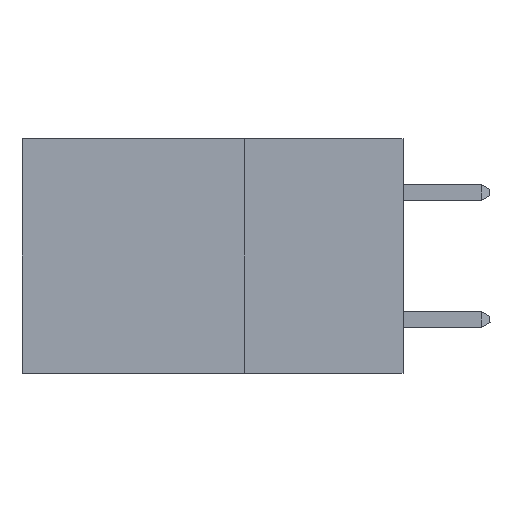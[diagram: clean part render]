
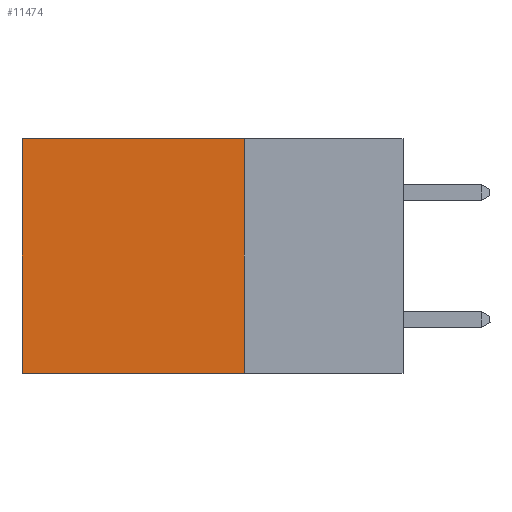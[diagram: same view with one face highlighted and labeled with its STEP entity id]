
A CAD part, left-side view. The second image highlights one B-rep face of the part: STEP entity #11474.
In plain terms, the highlighted planar face has unit normal (-1, 0, 0).
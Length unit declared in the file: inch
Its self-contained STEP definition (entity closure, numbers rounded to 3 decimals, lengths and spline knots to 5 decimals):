
#1245 = LINE ( 'NONE', #22937, #1663 ) ;
#1663 = VECTOR ( 'NONE', #23508, 39.37008 ) ;
#2475 = DIRECTION ( 'NONE',  ( 1., 0., 0. ) ) ;
#2815 = ORIENTED_EDGE ( 'NONE', *, *, #31033, .F. ) ;
#3150 = VECTOR ( 'NONE', #25215, 39.37008 ) ;
#3590 = VERTEX_POINT ( 'NONE', #11174 ) ;
#4204 = FACE_OUTER_BOUND ( 'NONE', #9429, .T. ) ;
#6728 = CARTESIAN_POINT ( 'NONE',  ( 0.2875, 0.25, -0.37 ) ) ;
#9253 = LINE ( 'NONE', #25268, #23292 ) ;
#9429 = EDGE_LOOP ( 'NONE', ( #11271, #14414, #2815, #14100 ) ) ;
#9713 = AXIS2_PLACEMENT_3D ( 'NONE', #24561, #2475, #12273 ) ;
#9776 = EDGE_CURVE ( 'NONE', #17253, #18858, #1245, .T. ) ;
#10226 = CARTESIAN_POINT ( 'NONE',  ( 0.2875, 0.25, 0. ) ) ;
#10698 = DIRECTION ( 'NONE',  ( 0., 1., 0. ) ) ;
#11025 = EDGE_CURVE ( 'NONE', #30353, #18858, #9253, .T. ) ;
#11174 = CARTESIAN_POINT ( 'NONE',  ( 0.2875, 0.25, 0. ) ) ;
#11271 = ORIENTED_EDGE ( 'NONE', *, *, #9776, .T. ) ;
#11344 = LINE ( 'NONE', #10226, #3150 ) ;
#11474 = ADVANCED_FACE ( 'NONE', ( #4204 ), #29878, .F. ) ;
#12273 = DIRECTION ( 'NONE',  ( 0., 0., -1. ) ) ;
#14100 = ORIENTED_EDGE ( 'NONE', *, *, #18255, .T. ) ;
#14414 = ORIENTED_EDGE ( 'NONE', *, *, #11025, .F. ) ;
#15604 = LINE ( 'NONE', #21056, #31131 ) ;
#17253 = VERTEX_POINT ( 'NONE', #22079 ) ;
#18255 = EDGE_CURVE ( 'NONE', #3590, #17253, #11344, .T. ) ;
#18858 = VERTEX_POINT ( 'NONE', #21833 ) ;
#21056 = CARTESIAN_POINT ( 'NONE',  ( 0.2875, 0.25, 0. ) ) ;
#21833 = CARTESIAN_POINT ( 'NONE',  ( 0.2875, 0.6, -0.37 ) ) ;
#22079 = CARTESIAN_POINT ( 'NONE',  ( 0.2875, 0.6, 0. ) ) ;
#22937 = CARTESIAN_POINT ( 'NONE',  ( 0.2875, 0.6, 0. ) ) ;
#23292 = VECTOR ( 'NONE', #10698, 39.37008 ) ;
#23508 = DIRECTION ( 'NONE',  ( 0., 0., -1. ) ) ;
#24561 = CARTESIAN_POINT ( 'NONE',  ( 0.2875, 0.25, 0. ) ) ;
#25215 = DIRECTION ( 'NONE',  ( 0., 1., 0. ) ) ;
#25268 = CARTESIAN_POINT ( 'NONE',  ( 0.2875, 0.25, -0.37 ) ) ;
#26276 = DIRECTION ( 'NONE',  ( 0., 0., -1. ) ) ;
#29878 = PLANE ( 'NONE',  #9713 ) ;
#30353 = VERTEX_POINT ( 'NONE', #6728 ) ;
#31033 = EDGE_CURVE ( 'NONE', #3590, #30353, #15604, .T. ) ;
#31131 = VECTOR ( 'NONE', #26276, 39.37008 ) ;
